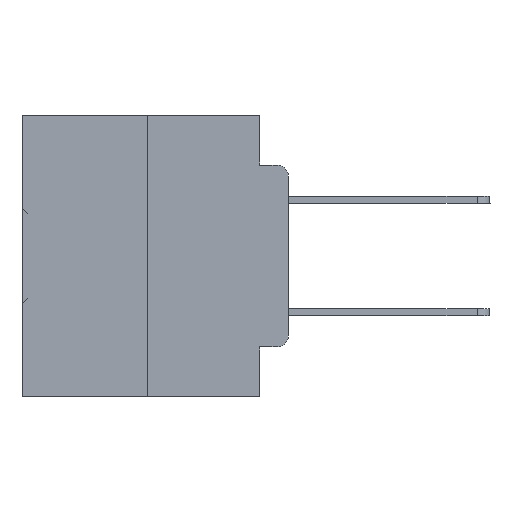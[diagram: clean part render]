
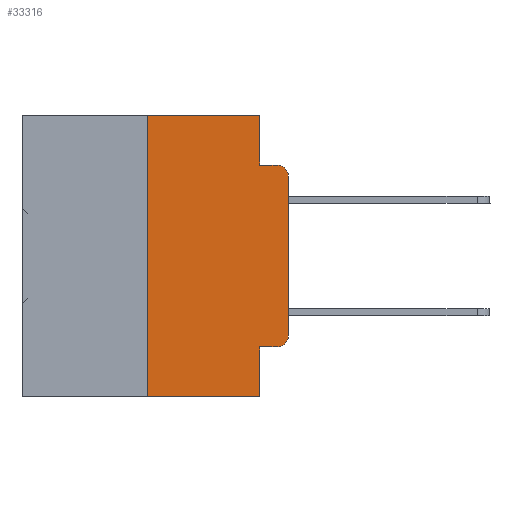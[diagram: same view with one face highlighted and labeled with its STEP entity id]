
A CAD part, left-side view. The second image highlights one B-rep face of the part: STEP entity #33316.
In plain terms, the highlighted planar face has unit normal (-1, 0, 0).
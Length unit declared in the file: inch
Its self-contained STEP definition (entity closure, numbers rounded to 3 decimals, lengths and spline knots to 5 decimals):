
#609 = CARTESIAN_POINT ( 'NONE',  ( 0., 0.051, 0. ) ) ;
#1580 = EDGE_CURVE ( 'NONE', #3353, #25416, #10202, .T. ) ;
#1687 = EDGE_LOOP ( 'NONE', ( #12490, #15513, #16952, #34386, #22809, #22710, #20374, #26459, #22565, #6282 ) ) ;
#2590 = EDGE_CURVE ( 'NONE', #31239, #33413, #10648, .T. ) ;
#2685 = DIRECTION ( 'NONE',  ( 0., -1., 0. ) ) ;
#2887 = CARTESIAN_POINT ( 'NONE',  ( 0., 0.051, -0.5 ) ) ;
#3353 = VERTEX_POINT ( 'NONE', #22045 ) ;
#3379 = VERTEX_POINT ( 'NONE', #26562 ) ;
#3502 = AXIS2_PLACEMENT_3D ( 'NONE', #11444, #5881, #22741 ) ;
#3692 = AXIS2_PLACEMENT_3D ( 'NONE', #10019, #3912, #21300 ) ;
#3803 = EDGE_CURVE ( 'NONE', #13721, #34990, #32386, .T. ) ;
#3912 = DIRECTION ( 'NONE',  ( -1., 0., 0. ) ) ;
#5881 = DIRECTION ( 'NONE',  ( -1., 0., 0. ) ) ;
#5979 = AXIS2_PLACEMENT_3D ( 'NONE', #22598, #13715, #7979 ) ;
#6270 = EDGE_CURVE ( 'NONE', #3353, #36004, #17463, .T. ) ;
#6282 = ORIENTED_EDGE ( 'NONE', *, *, #22375, .T. ) ;
#7502 = DIRECTION ( 'NONE',  ( 0., -1., 0. ) ) ;
#7634 = CIRCLE ( 'NONE', #3502, 0.02 ) ;
#7979 = DIRECTION ( 'NONE',  ( 0., 0., -1. ) ) ;
#8045 = LINE ( 'NONE', #32848, #13286 ) ;
#8194 = DIRECTION ( 'NONE',  ( 0., 0., 1. ) ) ;
#8658 = CARTESIAN_POINT ( 'NONE',  ( 0., 0., -0.3915 ) ) ;
#8744 = LINE ( 'NONE', #16886, #28145 ) ;
#9396 = DIRECTION ( 'NONE',  ( 0., -1., 0. ) ) ;
#9518 = EDGE_CURVE ( 'NONE', #16573, #31239, #20769, .T. ) ;
#10019 = CARTESIAN_POINT ( 'NONE',  ( 0., 0.02, -0.3915 ) ) ;
#10202 = LINE ( 'NONE', #32773, #33072 ) ;
#10648 = LINE ( 'NONE', #11208, #21299 ) ;
#11208 = CARTESIAN_POINT ( 'NONE',  ( 0., 0.051, -0.0885 ) ) ;
#11213 = EDGE_CURVE ( 'NONE', #3379, #25416, #28620, .T. ) ;
#11444 = CARTESIAN_POINT ( 'NONE',  ( 0., 0.02, -0.1085 ) ) ;
#12103 = DIRECTION ( 'NONE',  ( 0., -1., 0. ) ) ;
#12490 = ORIENTED_EDGE ( 'NONE', *, *, #3803, .T. ) ;
#12780 = VECTOR ( 'NONE', #12103, 39.37008 ) ;
#13267 = CARTESIAN_POINT ( 'NONE',  ( 0., 0.25, 0. ) ) ;
#13286 = VECTOR ( 'NONE', #7502, 39.37008 ) ;
#13715 = DIRECTION ( 'NONE',  ( 1., 0., 0. ) ) ;
#13721 = VERTEX_POINT ( 'NONE', #8658 ) ;
#14861 = DIRECTION ( 'NONE',  ( 0., 0., -1. ) ) ;
#15513 = ORIENTED_EDGE ( 'NONE', *, *, #18373, .T. ) ;
#16573 = VERTEX_POINT ( 'NONE', #25363 ) ;
#16859 = VECTOR ( 'NONE', #14861, 39.37008 ) ;
#16886 = CARTESIAN_POINT ( 'NONE',  ( 0., 0.25, 0. ) ) ;
#16952 = ORIENTED_EDGE ( 'NONE', *, *, #2590, .F. ) ;
#17463 = LINE ( 'NONE', #28752, #12780 ) ;
#18373 = EDGE_CURVE ( 'NONE', #34990, #33413, #7634, .T. ) ;
#19619 = FACE_OUTER_BOUND ( 'NONE', #1687, .T. ) ;
#20002 = CARTESIAN_POINT ( 'NONE',  ( 0., 0.02, -0.0885 ) ) ;
#20374 = ORIENTED_EDGE ( 'NONE', *, *, #11213, .T. ) ;
#20769 = LINE ( 'NONE', #609, #16859 ) ;
#21299 = VECTOR ( 'NONE', #2685, 39.37008 ) ;
#21300 = DIRECTION ( 'NONE',  ( 0., 0., -1. ) ) ;
#22023 = CIRCLE ( 'NONE', #3692, 0.02 ) ;
#22045 = CARTESIAN_POINT ( 'NONE',  ( 0., 0.051, -0.4115 ) ) ;
#22375 = EDGE_CURVE ( 'NONE', #36004, #13721, #22023, .T. ) ;
#22565 = ORIENTED_EDGE ( 'NONE', *, *, #6270, .T. ) ;
#22598 = CARTESIAN_POINT ( 'NONE',  ( 0., 0.473, 0. ) ) ;
#22710 = ORIENTED_EDGE ( 'NONE', *, *, #31830, .F. ) ;
#22741 = DIRECTION ( 'NONE',  ( 0., 0., -1. ) ) ;
#22809 = ORIENTED_EDGE ( 'NONE', *, *, #29857, .F. ) ;
#23279 = VECTOR ( 'NONE', #27364, 39.37008 ) ;
#25056 = CARTESIAN_POINT ( 'NONE',  ( 0., 0.02, -0.4115 ) ) ;
#25363 = CARTESIAN_POINT ( 'NONE',  ( 0., 0.051, 0. ) ) ;
#25416 = VERTEX_POINT ( 'NONE', #2887 ) ;
#25551 = PLANE ( 'NONE',  #5979 ) ;
#26459 = ORIENTED_EDGE ( 'NONE', *, *, #1580, .F. ) ;
#26562 = CARTESIAN_POINT ( 'NONE',  ( 0., 0.25, -0.5 ) ) ;
#27050 = DIRECTION ( 'NONE',  ( 0., 0., -1. ) ) ;
#27364 = DIRECTION ( 'NONE',  ( 0., 0., 1. ) ) ;
#27550 = CARTESIAN_POINT ( 'NONE',  ( 0., 0., -0.1085 ) ) ;
#28145 = VECTOR ( 'NONE', #8194, 39.37008 ) ;
#28620 = LINE ( 'NONE', #28971, #28747 ) ;
#28747 = VECTOR ( 'NONE', #9396, 39.37008 ) ;
#28752 = CARTESIAN_POINT ( 'NONE',  ( 0., 0.051, -0.4115 ) ) ;
#28971 = CARTESIAN_POINT ( 'NONE',  ( 0., 0.473, -0.5 ) ) ;
#29857 = EDGE_CURVE ( 'NONE', #32380, #16573, #8045, .T. ) ;
#30064 = CARTESIAN_POINT ( 'NONE',  ( 0., 0.051, -0.0885 ) ) ;
#31239 = VERTEX_POINT ( 'NONE', #30064 ) ;
#31830 = EDGE_CURVE ( 'NONE', #3379, #32380, #8744, .T. ) ;
#32380 = VERTEX_POINT ( 'NONE', #13267 ) ;
#32386 = LINE ( 'NONE', #32737, #23279 ) ;
#32737 = CARTESIAN_POINT ( 'NONE',  ( 0., 0., 0. ) ) ;
#32773 = CARTESIAN_POINT ( 'NONE',  ( 0., 0.051, 0. ) ) ;
#32848 = CARTESIAN_POINT ( 'NONE',  ( 0., 0.473, 0. ) ) ;
#33072 = VECTOR ( 'NONE', #27050, 39.37008 ) ;
#33316 = ADVANCED_FACE ( 'NONE', ( #19619 ), #25551, .F. ) ;
#33413 = VERTEX_POINT ( 'NONE', #20002 ) ;
#34386 = ORIENTED_EDGE ( 'NONE', *, *, #9518, .F. ) ;
#34990 = VERTEX_POINT ( 'NONE', #27550 ) ;
#36004 = VERTEX_POINT ( 'NONE', #25056 ) ;
